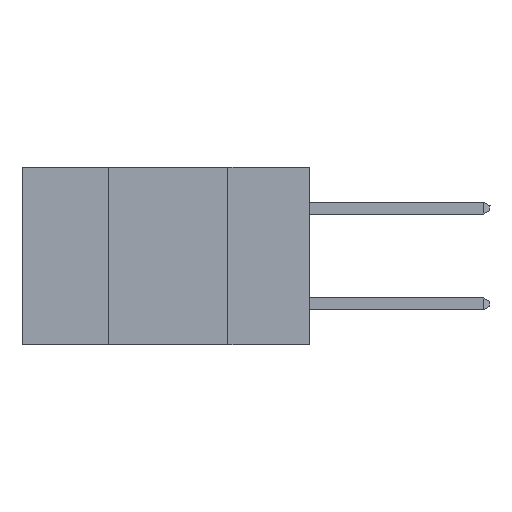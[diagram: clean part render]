
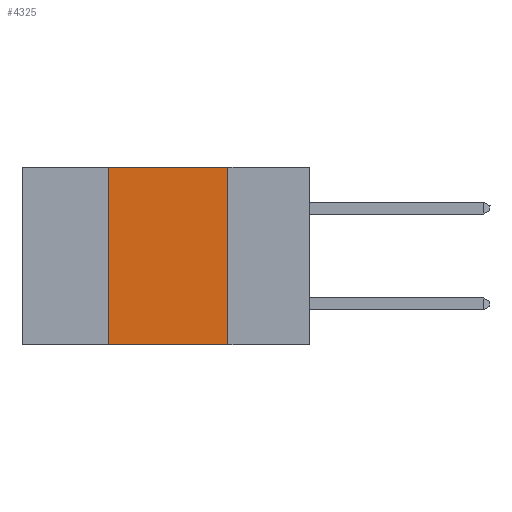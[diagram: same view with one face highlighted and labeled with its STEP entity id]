
A CAD part, left-side view. The second image highlights one B-rep face of the part: STEP entity #4325.
In plain terms, the highlighted planar face has unit normal (-1, 0, 0).
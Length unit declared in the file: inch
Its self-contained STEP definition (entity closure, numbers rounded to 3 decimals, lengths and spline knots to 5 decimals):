
#272 = VECTOR ( 'NONE', #11006, 39.37008 ) ;
#701 = AXIS2_PLACEMENT_3D ( 'NONE', #1687, #4877, #10715 ) ;
#935 = VERTEX_POINT ( 'NONE', #2264 ) ;
#1687 = CARTESIAN_POINT ( 'NONE',  ( 0., 0.6, 0. ) ) ;
#1796 = EDGE_CURVE ( 'NONE', #935, #2726, #9606, .T. ) ;
#2264 = CARTESIAN_POINT ( 'NONE',  ( 0., 0.42, 0. ) ) ;
#2542 = EDGE_CURVE ( 'NONE', #2726, #7171, #10802, .T. ) ;
#2575 = EDGE_CURVE ( 'NONE', #3817, #935, #8116, .T. ) ;
#2593 = EDGE_CURVE ( 'NONE', #3817, #7171, #10312, .T. ) ;
#2726 = VERTEX_POINT ( 'NONE', #10033 ) ;
#2924 = FACE_OUTER_BOUND ( 'NONE', #5656, .T. ) ;
#3817 = VERTEX_POINT ( 'NONE', #4415 ) ;
#3823 = PLANE ( 'NONE',  #701 ) ;
#4325 = ADVANCED_FACE ( 'NONE', ( #2924 ), #3823, .F. ) ;
#4415 = CARTESIAN_POINT ( 'NONE',  ( 0., 0.42, -0.37 ) ) ;
#4877 = DIRECTION ( 'NONE',  ( 1., 0., 0. ) ) ;
#5656 = EDGE_LOOP ( 'NONE', ( #11054, #11163, #11192, #11461 ) ) ;
#5960 = VECTOR ( 'NONE', #11172, 39.37008 ) ;
#6222 = VECTOR ( 'NONE', #11449, 39.37008 ) ;
#7171 = VERTEX_POINT ( 'NONE', #11644 ) ;
#7867 = CARTESIAN_POINT ( 'NONE',  ( 0., 0.6, 0. ) ) ;
#8095 = DIRECTION ( 'NONE',  ( 0., -1., 0. ) ) ;
#8116 = LINE ( 'NONE', #11198, #5960 ) ;
#9606 = LINE ( 'NONE', #7867, #11189 ) ;
#10033 = CARTESIAN_POINT ( 'NONE',  ( 0., 0.17, 0. ) ) ;
#10312 = LINE ( 'NONE', #11028, #272 ) ;
#10715 = DIRECTION ( 'NONE',  ( 0., 0., -1. ) ) ;
#10802 = LINE ( 'NONE', #11462, #6222 ) ;
#11006 = DIRECTION ( 'NONE',  ( 0., -1., 0. ) ) ;
#11028 = CARTESIAN_POINT ( 'NONE',  ( 0., 0.6, -0.37 ) ) ;
#11054 = ORIENTED_EDGE ( 'NONE', *, *, #2542, .F. ) ;
#11163 = ORIENTED_EDGE ( 'NONE', *, *, #1796, .F. ) ;
#11172 = DIRECTION ( 'NONE',  ( 0., 0., 1. ) ) ;
#11189 = VECTOR ( 'NONE', #8095, 39.37008 ) ;
#11192 = ORIENTED_EDGE ( 'NONE', *, *, #2575, .F. ) ;
#11198 = CARTESIAN_POINT ( 'NONE',  ( 0., 0.42, 0. ) ) ;
#11449 = DIRECTION ( 'NONE',  ( 0., 0., -1. ) ) ;
#11461 = ORIENTED_EDGE ( 'NONE', *, *, #2593, .T. ) ;
#11462 = CARTESIAN_POINT ( 'NONE',  ( 0., 0.17, 0. ) ) ;
#11644 = CARTESIAN_POINT ( 'NONE',  ( 0., 0.17, -0.37 ) ) ;
